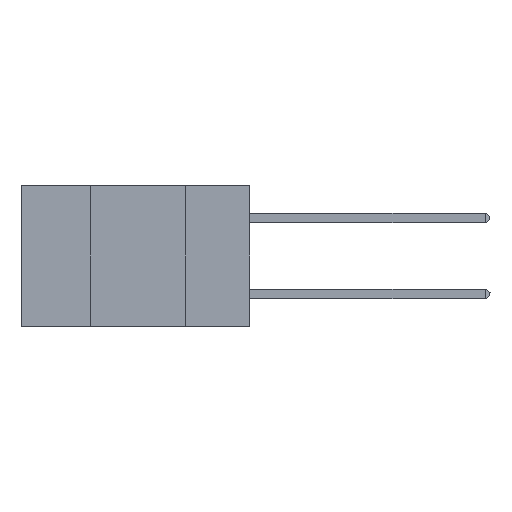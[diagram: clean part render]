
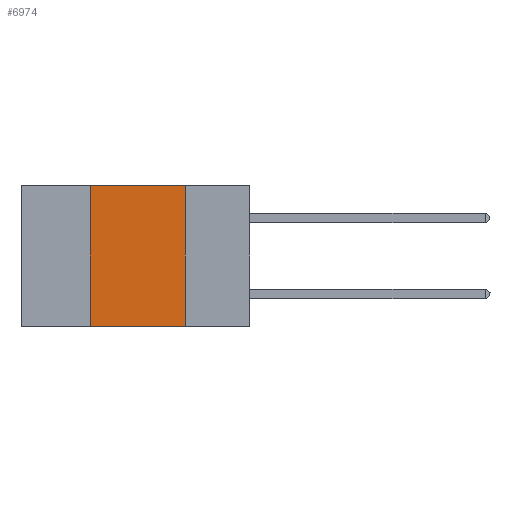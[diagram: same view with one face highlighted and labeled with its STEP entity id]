
A CAD part, left-side view. The second image highlights one B-rep face of the part: STEP entity #6974.
In plain terms, the highlighted planar face has unit normal (-1, 0, 0).
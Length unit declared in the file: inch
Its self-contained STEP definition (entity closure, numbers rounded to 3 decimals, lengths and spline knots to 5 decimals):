
#20 = DIRECTION ( 'NONE',  ( 0., 0., -1. ) ) ;
#1607 = PLANE ( 'NONE',  #16772 ) ;
#1857 = DIRECTION ( 'NONE',  ( 0., 0., 1. ) ) ;
#3597 = CARTESIAN_POINT ( 'NONE',  ( 0., 0.6, 0. ) ) ;
#5319 = EDGE_CURVE ( 'NONE', #9300, #19528, #19615, .T. ) ;
#6338 = CARTESIAN_POINT ( 'NONE',  ( 0., 0.42, -0.37 ) ) ;
#6586 = CARTESIAN_POINT ( 'NONE',  ( 0., 0.42, 0. ) ) ;
#6974 = ADVANCED_FACE ( 'NONE', ( #18348 ), #1607, .F. ) ;
#8728 = DIRECTION ( 'NONE',  ( 0., -1., 0. ) ) ;
#9202 = DIRECTION ( 'NONE',  ( 1., 0., 0. ) ) ;
#9300 = VERTEX_POINT ( 'NONE', #6338 ) ;
#10311 = LINE ( 'NONE', #20331, #14514 ) ;
#11058 = ORIENTED_EDGE ( 'NONE', *, *, #13878, .F. ) ;
#12993 = ORIENTED_EDGE ( 'NONE', *, *, #5319, .F. ) ;
#13129 = CARTESIAN_POINT ( 'NONE',  ( 0., 0.6, 0. ) ) ;
#13562 = VECTOR ( 'NONE', #24070, 39.37008 ) ;
#13878 = EDGE_CURVE ( 'NONE', #19939, #21895, #10311, .T. ) ;
#14514 = VECTOR ( 'NONE', #17811, 39.37008 ) ;
#14526 = VECTOR ( 'NONE', #8728, 39.37008 ) ;
#15185 = ORIENTED_EDGE ( 'NONE', *, *, #18675, .F. ) ;
#16772 = AXIS2_PLACEMENT_3D ( 'NONE', #13129, #9202, #20 ) ;
#17196 = LINE ( 'NONE', #21854, #14526 ) ;
#17299 = CARTESIAN_POINT ( 'NONE',  ( 0., 0.17, 0. ) ) ;
#17811 = DIRECTION ( 'NONE',  ( 0., 0., -1. ) ) ;
#18348 = FACE_OUTER_BOUND ( 'NONE', #21598, .T. ) ;
#18408 = VECTOR ( 'NONE', #1857, 39.37008 ) ;
#18675 = EDGE_CURVE ( 'NONE', #19528, #19939, #21224, .T. ) ;
#19528 = VERTEX_POINT ( 'NONE', #6586 ) ;
#19615 = LINE ( 'NONE', #21703, #18408 ) ;
#19939 = VERTEX_POINT ( 'NONE', #17299 ) ;
#20331 = CARTESIAN_POINT ( 'NONE',  ( 0., 0.17, 0. ) ) ;
#21224 = LINE ( 'NONE', #3597, #13562 ) ;
#21598 = EDGE_LOOP ( 'NONE', ( #11058, #15185, #12993, #24304 ) ) ;
#21703 = CARTESIAN_POINT ( 'NONE',  ( 0., 0.42, 0. ) ) ;
#21854 = CARTESIAN_POINT ( 'NONE',  ( 0., 0.6, -0.37 ) ) ;
#21858 = CARTESIAN_POINT ( 'NONE',  ( 0., 0.17, -0.37 ) ) ;
#21895 = VERTEX_POINT ( 'NONE', #21858 ) ;
#23111 = EDGE_CURVE ( 'NONE', #9300, #21895, #17196, .T. ) ;
#24070 = DIRECTION ( 'NONE',  ( 0., -1., 0. ) ) ;
#24304 = ORIENTED_EDGE ( 'NONE', *, *, #23111, .T. ) ;
